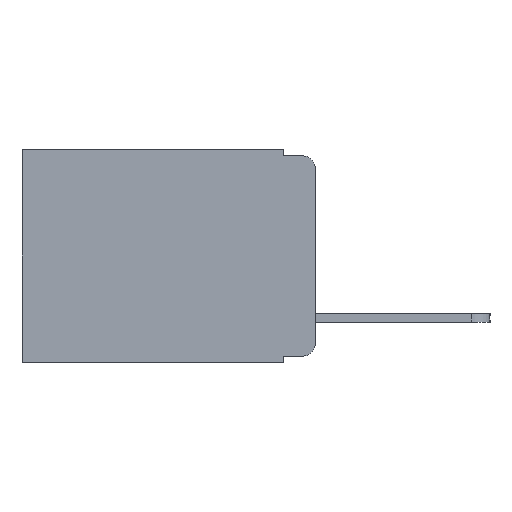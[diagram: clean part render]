
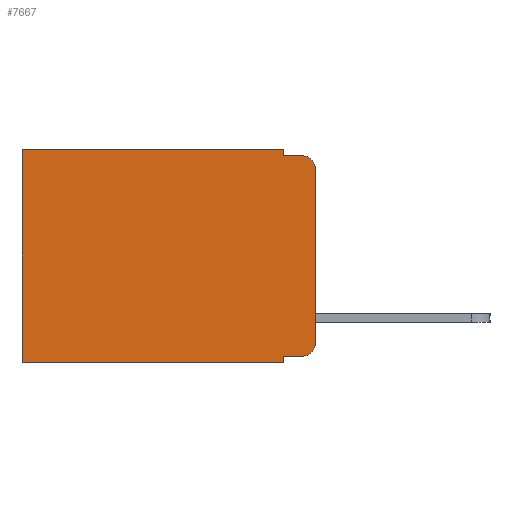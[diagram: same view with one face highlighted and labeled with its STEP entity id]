
A CAD part, left-side view. The second image highlights one B-rep face of the part: STEP entity #7667.
In plain terms, the highlighted planar face has unit normal (-1, 0, 0).
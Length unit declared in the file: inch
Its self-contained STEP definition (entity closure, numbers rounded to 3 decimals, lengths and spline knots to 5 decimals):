
#120 = CARTESIAN_POINT ( 'NONE',  ( 0.298, 0.051, 0. ) ) ;
#162 = PLANE ( 'NONE',  #5402 ) ;
#312 = VERTEX_POINT ( 'NONE', #1860 ) ;
#591 = DIRECTION ( 'NONE',  ( -1., 0., 0. ) ) ;
#627 = CARTESIAN_POINT ( 'NONE',  ( 0.298, 0.051, -0.333 ) ) ;
#733 = VERTEX_POINT ( 'NONE', #120 ) ;
#901 = CARTESIAN_POINT ( 'NONE',  ( 0.298, 0., 0. ) ) ;
#1110 = CARTESIAN_POINT ( 'NONE',  ( 0.298, 0.051, -0.01 ) ) ;
#1250 = LINE ( 'NONE', #10765, #11015 ) ;
#1356 = EDGE_CURVE ( 'NONE', #733, #10753, #9337, .T. ) ;
#1574 = EDGE_CURVE ( 'NONE', #10753, #11452, #7138, .T. ) ;
#1632 = LINE ( 'NONE', #8209, #6486 ) ;
#1651 = CARTESIAN_POINT ( 'NONE',  ( 0.298, 0., -0.03 ) ) ;
#1860 = CARTESIAN_POINT ( 'NONE',  ( 0.298, 0.051, -0.343 ) ) ;
#2236 = CARTESIAN_POINT ( 'NONE',  ( 0.298, 0.02, -0.01 ) ) ;
#2320 = CARTESIAN_POINT ( 'NONE',  ( 0.298, 0.473, -0.343 ) ) ;
#2346 = VERTEX_POINT ( 'NONE', #9929 ) ;
#2436 = DIRECTION ( 'NONE',  ( 0., 0., -1. ) ) ;
#2460 = VECTOR ( 'NONE', #10962, 39.37008 ) ;
#2572 = CARTESIAN_POINT ( 'NONE',  ( 0.298, 0.473, 0. ) ) ;
#2603 = ORIENTED_EDGE ( 'NONE', *, *, #6226, .T. ) ;
#2650 = VERTEX_POINT ( 'NONE', #10050 ) ;
#2734 = DIRECTION ( 'NONE',  ( 0., 0., -1. ) ) ;
#2877 = CARTESIAN_POINT ( 'NONE',  ( 0.298, 0., 0. ) ) ;
#2933 = ORIENTED_EDGE ( 'NONE', *, *, #5610, .T. ) ;
#3044 = VERTEX_POINT ( 'NONE', #627 ) ;
#3094 = DIRECTION ( 'NONE',  ( 1., 0., 0. ) ) ;
#4054 = ORIENTED_EDGE ( 'NONE', *, *, #1574, .F. ) ;
#4088 = DIRECTION ( 'NONE',  ( 0., 0., -1. ) ) ;
#4259 = DIRECTION ( 'NONE',  ( 0., -1., 0. ) ) ;
#4367 = CIRCLE ( 'NONE', #11309, 0.02 ) ;
#4370 = DIRECTION ( 'NONE',  ( 0., 0., -1. ) ) ;
#4391 = ORIENTED_EDGE ( 'NONE', *, *, #11231, .T. ) ;
#4818 = VECTOR ( 'NONE', #11478, 39.37008 ) ;
#5050 = VECTOR ( 'NONE', #4259, 39.37008 ) ;
#5084 = LINE ( 'NONE', #10620, #4818 ) ;
#5402 = AXIS2_PLACEMENT_3D ( 'NONE', #901, #3094, #4088 ) ;
#5417 = VECTOR ( 'NONE', #6412, 39.37008 ) ;
#5610 = EDGE_CURVE ( 'NONE', #2346, #2650, #4367, .T. ) ;
#5737 = FACE_OUTER_BOUND ( 'NONE', #9739, .T. ) ;
#5875 = VERTEX_POINT ( 'NONE', #1651 ) ;
#5926 = ORIENTED_EDGE ( 'NONE', *, *, #7323, .F. ) ;
#6166 = CARTESIAN_POINT ( 'NONE',  ( 0.298, 0.051, 0. ) ) ;
#6226 = EDGE_CURVE ( 'NONE', #3044, #2346, #5084, .T. ) ;
#6412 = DIRECTION ( 'NONE',  ( 0., 0., -1. ) ) ;
#6452 = VECTOR ( 'NONE', #2436, 39.37008 ) ;
#6457 = VERTEX_POINT ( 'NONE', #9601 ) ;
#6486 = VECTOR ( 'NONE', #2734, 39.37008 ) ;
#6516 = VERTEX_POINT ( 'NONE', #2320 ) ;
#6828 = EDGE_CURVE ( 'NONE', #3044, #312, #1632, .T. ) ;
#6887 = LINE ( 'NONE', #10329, #7156 ) ;
#7138 = LINE ( 'NONE', #8282, #5050 ) ;
#7156 = VECTOR ( 'NONE', #9819, 39.37008 ) ;
#7323 = EDGE_CURVE ( 'NONE', #5875, #2650, #1250, .T. ) ;
#7357 = ORIENTED_EDGE ( 'NONE', *, *, #7516, .F. ) ;
#7516 = EDGE_CURVE ( 'NONE', #312, #6516, #6887, .T. ) ;
#7667 = ADVANCED_FACE ( 'NONE', ( #5737 ), #162, .F. ) ;
#7845 = LINE ( 'NONE', #2572, #5417 ) ;
#8209 = CARTESIAN_POINT ( 'NONE',  ( 0.298, 0.051, 0. ) ) ;
#8282 = CARTESIAN_POINT ( 'NONE',  ( 0.298, 0.051, -0.01 ) ) ;
#8382 = DIRECTION ( 'NONE',  ( 0., 0., -1. ) ) ;
#8891 = ORIENTED_EDGE ( 'NONE', *, *, #9497, .T. ) ;
#9337 = LINE ( 'NONE', #6166, #6452 ) ;
#9497 = EDGE_CURVE ( 'NONE', #5875, #11452, #9572, .T. ) ;
#9572 = CIRCLE ( 'NONE', #9824, 0.02 ) ;
#9601 = CARTESIAN_POINT ( 'NONE',  ( 0.298, 0.473, 0. ) ) ;
#9739 = EDGE_LOOP ( 'NONE', ( #5926, #8891, #4054, #11577, #4391, #11844, #7357, #9904, #2603, #2933 ) ) ;
#9793 = LINE ( 'NONE', #2877, #2460 ) ;
#9819 = DIRECTION ( 'NONE',  ( 0., 1., 0. ) ) ;
#9824 = AXIS2_PLACEMENT_3D ( 'NONE', #10170, #10102, #10076 ) ;
#9867 = CARTESIAN_POINT ( 'NONE',  ( 0.298, 0.02, -0.313 ) ) ;
#9904 = ORIENTED_EDGE ( 'NONE', *, *, #6828, .F. ) ;
#9929 = CARTESIAN_POINT ( 'NONE',  ( 0.298, 0.02, -0.333 ) ) ;
#10050 = CARTESIAN_POINT ( 'NONE',  ( 0.298, 0., -0.313 ) ) ;
#10076 = DIRECTION ( 'NONE',  ( 0., 0., -1. ) ) ;
#10102 = DIRECTION ( 'NONE',  ( -1., 0., 0. ) ) ;
#10170 = CARTESIAN_POINT ( 'NONE',  ( 0.298, 0.02, -0.03 ) ) ;
#10286 = EDGE_CURVE ( 'NONE', #6457, #6516, #7845, .T. ) ;
#10329 = CARTESIAN_POINT ( 'NONE',  ( 0.298, 0., -0.343 ) ) ;
#10620 = CARTESIAN_POINT ( 'NONE',  ( 0.298, 0.051, -0.333 ) ) ;
#10753 = VERTEX_POINT ( 'NONE', #1110 ) ;
#10765 = CARTESIAN_POINT ( 'NONE',  ( 0.298, 0., 0. ) ) ;
#10962 = DIRECTION ( 'NONE',  ( 0., 1., 0. ) ) ;
#11015 = VECTOR ( 'NONE', #8382, 39.37008 ) ;
#11231 = EDGE_CURVE ( 'NONE', #733, #6457, #9793, .T. ) ;
#11309 = AXIS2_PLACEMENT_3D ( 'NONE', #9867, #591, #4370 ) ;
#11452 = VERTEX_POINT ( 'NONE', #2236 ) ;
#11478 = DIRECTION ( 'NONE',  ( 0., -1., 0. ) ) ;
#11577 = ORIENTED_EDGE ( 'NONE', *, *, #1356, .F. ) ;
#11844 = ORIENTED_EDGE ( 'NONE', *, *, #10286, .T. ) ;
